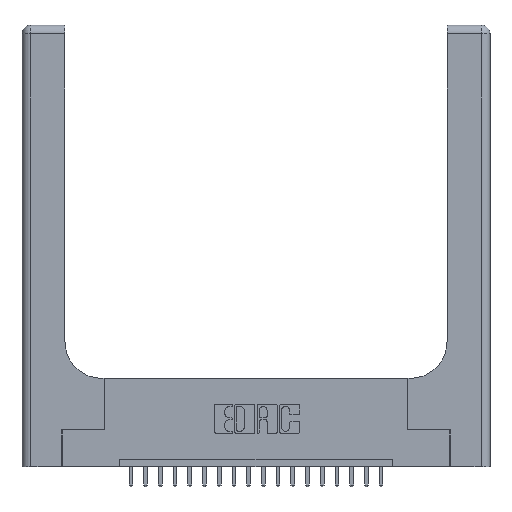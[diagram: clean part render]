
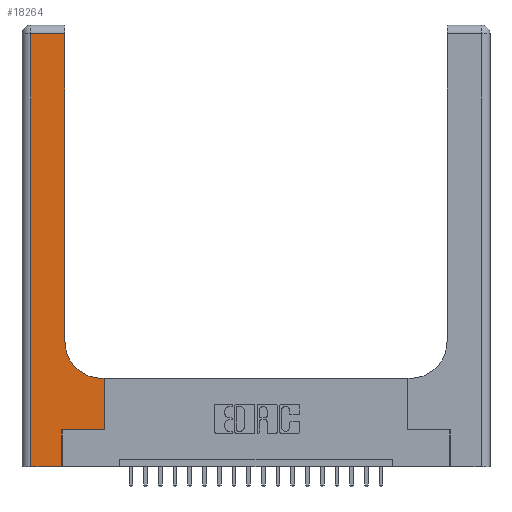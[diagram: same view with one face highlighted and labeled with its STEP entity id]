
A CAD part, top view. The second image highlights one B-rep face of the part: STEP entity #18264.
In plain terms, the highlighted planar face has unit normal (0, 0, 1).
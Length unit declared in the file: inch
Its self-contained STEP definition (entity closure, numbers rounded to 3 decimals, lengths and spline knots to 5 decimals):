
#77 = LINE ( 'NONE', #7717, #11775 ) ;
#507 = LINE ( 'NONE', #8362, #6138 ) ;
#920 = CARTESIAN_POINT ( 'NONE',  ( 0.5585, 0.6, 0.37 ) ) ;
#1146 = DIRECTION ( 'NONE',  ( 0., 1., 0. ) ) ;
#1411 = ORIENTED_EDGE ( 'NONE', *, *, #21919, .T. ) ;
#1710 = VECTOR ( 'NONE', #8777, 39.37008 ) ;
#1729 = CARTESIAN_POINT ( 'NONE',  ( 0.2915, 0.85, 0.37 ) ) ;
#1849 = EDGE_CURVE ( 'NONE', #13783, #3164, #14367, .T. ) ;
#1967 = VERTEX_POINT ( 'NONE', #17717 ) ;
#2054 = AXIS2_PLACEMENT_3D ( 'NONE', #19291, #14053, #12299 ) ;
#2200 = DIRECTION ( 'NONE',  ( 1., 0., 0. ) ) ;
#2598 = VERTEX_POINT ( 'NONE', #14387 ) ;
#3066 = DIRECTION ( 'NONE',  ( 0., -1., 0. ) ) ;
#3085 = CARTESIAN_POINT ( 'NONE',  ( 0.269, 0.25, 0.37 ) ) ;
#3150 = VERTEX_POINT ( 'NONE', #11102 ) ;
#3164 = VERTEX_POINT ( 'NONE', #920 ) ;
#3547 = LINE ( 'NONE', #11547, #6441 ) ;
#3565 = EDGE_CURVE ( 'NONE', #3164, #1967, #507, .T. ) ;
#3603 = ORIENTED_EDGE ( 'NONE', *, *, #13372, .T. ) ;
#3650 = CIRCLE ( 'NONE', #17656, 0.25 ) ;
#4262 = DIRECTION ( 'NONE',  ( -1., 0., 0. ) ) ;
#6138 = VECTOR ( 'NONE', #16590, 39.37008 ) ;
#6441 = VECTOR ( 'NONE', #3066, 39.37008 ) ;
#6797 = LINE ( 'NONE', #21072, #18125 ) ;
#6925 = ORIENTED_EDGE ( 'NONE', *, *, #21292, .T. ) ;
#7142 = CARTESIAN_POINT ( 'NONE',  ( 0.269, 0.25, 0.37 ) ) ;
#7717 = CARTESIAN_POINT ( 'NONE',  ( 0.269, 0., 0.37 ) ) ;
#8068 = ORIENTED_EDGE ( 'NONE', *, *, #16113, .T. ) ;
#8362 = CARTESIAN_POINT ( 'NONE',  ( 0.2915, 0.6, 0.37 ) ) ;
#8777 = DIRECTION ( 'NONE',  ( 0., 1., 0. ) ) ;
#8906 = ORIENTED_EDGE ( 'NONE', *, *, #3565, .T. ) ;
#9053 = EDGE_LOOP ( 'NONE', ( #11904, #16941, #20157, #1411, #8068, #3603, #15014, #8906, #6925 ) ) ;
#9136 = PLANE ( 'NONE',  #2054 ) ;
#9795 = VERTEX_POINT ( 'NONE', #21132 ) ;
#10088 = DIRECTION ( 'NONE',  ( 1., 0., 0. ) ) ;
#11102 = CARTESIAN_POINT ( 'NONE',  ( 0.06, 0., 0.37 ) ) ;
#11547 = CARTESIAN_POINT ( 'NONE',  ( 0.06, 3., 0.37 ) ) ;
#11775 = VECTOR ( 'NONE', #1146, 39.37008 ) ;
#11904 = ORIENTED_EDGE ( 'NONE', *, *, #16585, .T. ) ;
#11996 = FACE_OUTER_BOUND ( 'NONE', #9053, .T. ) ;
#12054 = CARTESIAN_POINT ( 'NONE',  ( 0.06, 2.94, 0.37 ) ) ;
#12187 = VERTEX_POINT ( 'NONE', #12054 ) ;
#12299 = DIRECTION ( 'NONE',  ( -1., 0., 0. ) ) ;
#12553 = VECTOR ( 'NONE', #15770, 39.37008 ) ;
#13182 = VECTOR ( 'NONE', #2200, 39.37008 ) ;
#13372 = EDGE_CURVE ( 'NONE', #14569, #13783, #16069, .T. ) ;
#13783 = VERTEX_POINT ( 'NONE', #14615 ) ;
#14019 = CARTESIAN_POINT ( 'NONE',  ( 0.5585, 0.25, 0.37 ) ) ;
#14053 = DIRECTION ( 'NONE',  ( 0., 0., -1. ) ) ;
#14367 = LINE ( 'NONE', #14019, #12553 ) ;
#14387 = CARTESIAN_POINT ( 'NONE',  ( 0.269, 0., 0.37 ) ) ;
#14544 = LINE ( 'NONE', #15994, #18525 ) ;
#14569 = VERTEX_POINT ( 'NONE', #7142 ) ;
#14615 = CARTESIAN_POINT ( 'NONE',  ( 0.5585, 0.25, 0.37 ) ) ;
#15014 = ORIENTED_EDGE ( 'NONE', *, *, #1849, .T. ) ;
#15147 = CARTESIAN_POINT ( 'NONE',  ( 0.5415, 0.85, 0.37 ) ) ;
#15770 = DIRECTION ( 'NONE',  ( 0., 1., 0. ) ) ;
#15994 = CARTESIAN_POINT ( 'NONE',  ( 0., 2.94, 0.37 ) ) ;
#16069 = LINE ( 'NONE', #3085, #13182 ) ;
#16113 = EDGE_CURVE ( 'NONE', #2598, #14569, #77, .T. ) ;
#16585 = EDGE_CURVE ( 'NONE', #17697, #9795, #18089, .T. ) ;
#16590 = DIRECTION ( 'NONE',  ( -1., 0., 0. ) ) ;
#16941 = ORIENTED_EDGE ( 'NONE', *, *, #19547, .T. ) ;
#17648 = EDGE_CURVE ( 'NONE', #12187, #3150, #3547, .T. ) ;
#17656 = AXIS2_PLACEMENT_3D ( 'NONE', #15147, #20193, #10088 ) ;
#17697 = VERTEX_POINT ( 'NONE', #1729 ) ;
#17717 = CARTESIAN_POINT ( 'NONE',  ( 0.5415, 0.6, 0.37 ) ) ;
#17720 = DIRECTION ( 'NONE',  ( 1., 0., 0. ) ) ;
#18089 = LINE ( 'NONE', #19163, #1710 ) ;
#18125 = VECTOR ( 'NONE', #17720, 39.37008 ) ;
#18264 = ADVANCED_FACE ( 'NONE', ( #11996 ), #9136, .F. ) ;
#18525 = VECTOR ( 'NONE', #4262, 39.37008 ) ;
#19163 = CARTESIAN_POINT ( 'NONE',  ( 0.2915, 3., 0.37 ) ) ;
#19291 = CARTESIAN_POINT ( 'NONE',  ( 0., 3., 0.37 ) ) ;
#19547 = EDGE_CURVE ( 'NONE', #9795, #12187, #14544, .T. ) ;
#20157 = ORIENTED_EDGE ( 'NONE', *, *, #17648, .T. ) ;
#20193 = DIRECTION ( 'NONE',  ( 0., 0., -1. ) ) ;
#21072 = CARTESIAN_POINT ( 'NONE',  ( 0., 0., 0.37 ) ) ;
#21132 = CARTESIAN_POINT ( 'NONE',  ( 0.2915, 2.94, 0.37 ) ) ;
#21292 = EDGE_CURVE ( 'NONE', #1967, #17697, #3650, .T. ) ;
#21919 = EDGE_CURVE ( 'NONE', #3150, #2598, #6797, .T. ) ;
